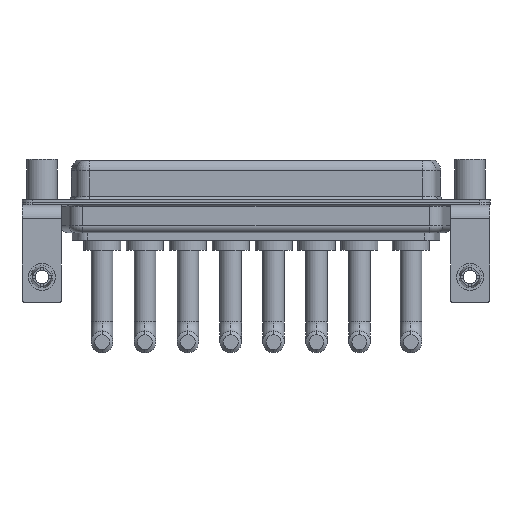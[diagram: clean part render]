
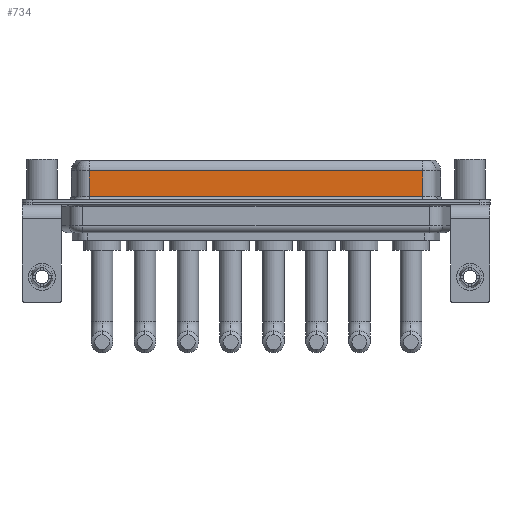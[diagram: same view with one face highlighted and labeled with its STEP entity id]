
A CAD part, front view. The second image highlights one B-rep face of the part: STEP entity #734.
In plain terms, the highlighted planar face has unit normal (0, -1, 0).
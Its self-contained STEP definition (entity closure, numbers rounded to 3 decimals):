
#734 = ADVANCED_FACE ( 'NONE', ( #7640 ), #13949, .F. ) ;
#984 = LINE ( 'NONE', #10294, #10862 ) ;
#1076 = DIRECTION ( 'NONE',  ( 0., 0., -1. ) ) ;
#1164 = DIRECTION ( 'NONE',  ( 0., 1., 0. ) ) ;
#1226 = CARTESIAN_POINT ( 'NONE',  ( 56.462, -3.95, 0.9 ) ) ;
#1491 = ORIENTED_EDGE ( 'NONE', *, *, #9406, .F. ) ;
#2169 = VECTOR ( 'NONE', #6417, 1000. ) ;
#2985 = VERTEX_POINT ( 'NONE', #16698 ) ;
#3565 = DIRECTION ( 'NONE',  ( 0., 0., -1. ) ) ;
#3895 = ORIENTED_EDGE ( 'NONE', *, *, #5433, .T. ) ;
#4904 = CARTESIAN_POINT ( 'NONE',  ( 56.462, -3.95, 6.4 ) ) ;
#4974 = VERTEX_POINT ( 'NONE', #8879 ) ;
#5433 = EDGE_CURVE ( 'NONE', #16121, #4974, #9037, .T. ) ;
#6381 = DIRECTION ( 'NONE',  ( -1., 0., 0. ) ) ;
#6417 = DIRECTION ( 'NONE',  ( 1., 0., 0. ) ) ;
#6422 = CARTESIAN_POINT ( 'NONE',  ( 56.462, -3.95, 4.65 ) ) ;
#6496 = ORIENTED_EDGE ( 'NONE', *, *, #8513, .T. ) ;
#7640 = FACE_OUTER_BOUND ( 'NONE', #10886, .T. ) ;
#8513 = EDGE_CURVE ( 'NONE', #4974, #2985, #984, .T. ) ;
#8879 = CARTESIAN_POINT ( 'NONE',  ( 7.038, -3.95, 4.65 ) ) ;
#9037 = LINE ( 'NONE', #16678, #10822 ) ;
#9406 = EDGE_CURVE ( 'NONE', #16121, #13485, #9813, .T. ) ;
#9813 = LINE ( 'NONE', #12615, #11386 ) ;
#10294 = CARTESIAN_POINT ( 'NONE',  ( 7.038, -3.95, 6.4 ) ) ;
#10738 = ORIENTED_EDGE ( 'NONE', *, *, #13788, .T. ) ;
#10798 = CARTESIAN_POINT ( 'NONE',  ( 56.462, -3.95, 0.9 ) ) ;
#10822 = VECTOR ( 'NONE', #6381, 1000. ) ;
#10862 = VECTOR ( 'NONE', #1076, 1000. ) ;
#10886 = EDGE_LOOP ( 'NONE', ( #1491, #3895, #6496, #10738 ) ) ;
#11386 = VECTOR ( 'NONE', #3565, 1000. ) ;
#12568 = AXIS2_PLACEMENT_3D ( 'NONE', #4904, #1164, #12929 ) ;
#12615 = CARTESIAN_POINT ( 'NONE',  ( 56.462, -3.95, 6.4 ) ) ;
#12911 = LINE ( 'NONE', #1226, #2169 ) ;
#12929 = DIRECTION ( 'NONE',  ( 0., 0., 1. ) ) ;
#13485 = VERTEX_POINT ( 'NONE', #10798 ) ;
#13788 = EDGE_CURVE ( 'NONE', #2985, #13485, #12911, .T. ) ;
#13949 = PLANE ( 'NONE',  #12568 ) ;
#16121 = VERTEX_POINT ( 'NONE', #6422 ) ;
#16678 = CARTESIAN_POINT ( 'NONE',  ( 56.462, -3.95, 4.65 ) ) ;
#16698 = CARTESIAN_POINT ( 'NONE',  ( 7.038, -3.95, 0.9 ) ) ;
